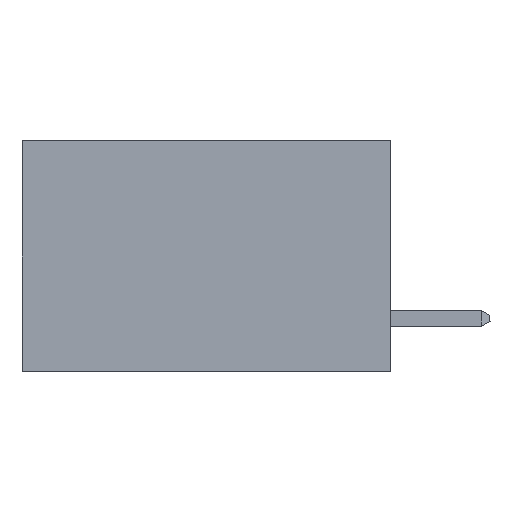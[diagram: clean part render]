
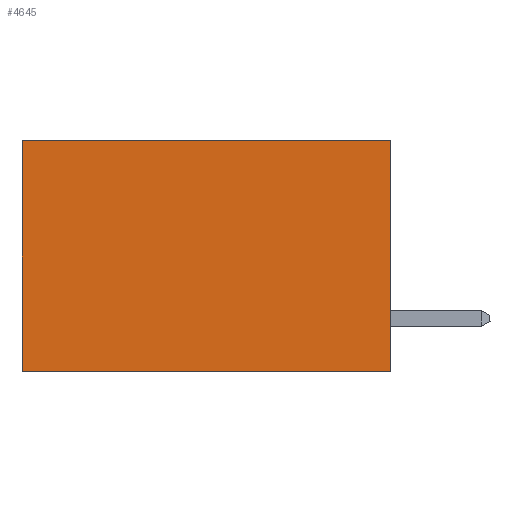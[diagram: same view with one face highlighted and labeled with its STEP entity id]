
A CAD part, left-side view. The second image highlights one B-rep face of the part: STEP entity #4645.
In plain terms, the highlighted planar face has unit normal (-1, 0, 0).
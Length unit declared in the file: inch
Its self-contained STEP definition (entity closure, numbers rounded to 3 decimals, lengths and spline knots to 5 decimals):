
#23 = CARTESIAN_POINT ( 'NONE',  ( 0.277, 0., 0. ) ) ;
#260 = EDGE_CURVE ( 'NONE', #3426, #5098, #5199, .T. ) ;
#303 = EDGE_CURVE ( 'NONE', #5098, #3455, #8195, .T. ) ;
#418 = AXIS2_PLACEMENT_3D ( 'NONE', #1357, #16410, #13290 ) ;
#987 = ORIENTED_EDGE ( 'NONE', *, *, #303, .F. ) ;
#1357 = CARTESIAN_POINT ( 'NONE',  ( 0.277, 0., -0.37 ) ) ;
#1759 = VECTOR ( 'NONE', #14406, 39.37008 ) ;
#2189 = LINE ( 'NONE', #12761, #6411 ) ;
#3426 = VERTEX_POINT ( 'NONE', #23 ) ;
#3455 = VERTEX_POINT ( 'NONE', #9340 ) ;
#4413 = ORIENTED_EDGE ( 'NONE', *, *, #260, .F. ) ;
#4644 = CARTESIAN_POINT ( 'NONE',  ( 0.277, 0., -0.37 ) ) ;
#4645 = ADVANCED_FACE ( 'NONE', ( #5401 ), #9815, .F. ) ;
#5098 = VERTEX_POINT ( 'NONE', #4644 ) ;
#5111 = DIRECTION ( 'NONE',  ( 0., 1., 0. ) ) ;
#5138 = EDGE_CURVE ( 'NONE', #6445, #3455, #14835, .T. ) ;
#5199 = LINE ( 'NONE', #13959, #1759 ) ;
#5224 = ORIENTED_EDGE ( 'NONE', *, *, #15987, .T. ) ;
#5401 = FACE_OUTER_BOUND ( 'NONE', #16253, .T. ) ;
#6411 = VECTOR ( 'NONE', #5111, 39.37008 ) ;
#6445 = VERTEX_POINT ( 'NONE', #6775 ) ;
#6775 = CARTESIAN_POINT ( 'NONE',  ( 0.277, 0.59, 0. ) ) ;
#7793 = VECTOR ( 'NONE', #10482, 39.37008 ) ;
#8195 = LINE ( 'NONE', #14546, #7793 ) ;
#9340 = CARTESIAN_POINT ( 'NONE',  ( 0.277, 0.59, -0.37 ) ) ;
#9815 = PLANE ( 'NONE',  #418 ) ;
#10482 = DIRECTION ( 'NONE',  ( 0., 1., 0. ) ) ;
#11200 = DIRECTION ( 'NONE',  ( 0., 0., -1. ) ) ;
#12680 = CARTESIAN_POINT ( 'NONE',  ( 0.277, 0.59, -0.37 ) ) ;
#12761 = CARTESIAN_POINT ( 'NONE',  ( 0.277, 0., 0. ) ) ;
#13290 = DIRECTION ( 'NONE',  ( 0., 0., -1. ) ) ;
#13845 = ORIENTED_EDGE ( 'NONE', *, *, #5138, .T. ) ;
#13959 = CARTESIAN_POINT ( 'NONE',  ( 0.277, 0., -0.37 ) ) ;
#14406 = DIRECTION ( 'NONE',  ( 0., 0., -1. ) ) ;
#14410 = VECTOR ( 'NONE', #11200, 39.37008 ) ;
#14546 = CARTESIAN_POINT ( 'NONE',  ( 0.277, 0., -0.37 ) ) ;
#14835 = LINE ( 'NONE', #12680, #14410 ) ;
#15987 = EDGE_CURVE ( 'NONE', #3426, #6445, #2189, .T. ) ;
#16253 = EDGE_LOOP ( 'NONE', ( #13845, #987, #4413, #5224 ) ) ;
#16410 = DIRECTION ( 'NONE',  ( 1., 0., 0. ) ) ;
